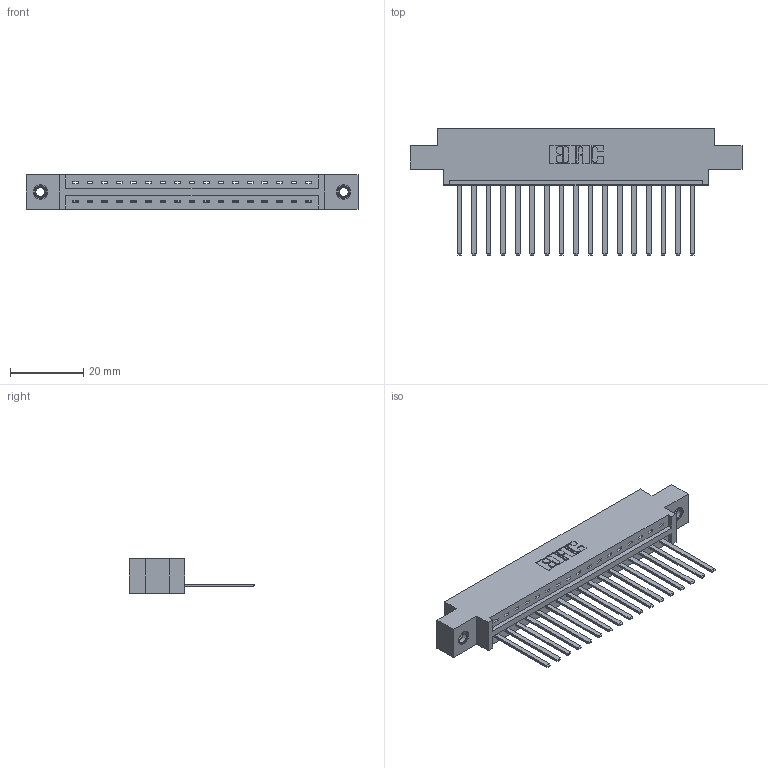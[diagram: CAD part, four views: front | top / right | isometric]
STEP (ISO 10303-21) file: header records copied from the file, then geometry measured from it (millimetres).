
FILE_DESCRIPTION (( 'STEP AP203' ), '1' );
FILE_NAME ('337-017-544-607.STEP', '2018-08-04T22:29:34', ( '' ), ( '' ), 'SwSTEP 2.0', 'SolidWorks 2016', '' );
FILE_SCHEMA (( 'CONFIG_CONTROL_DESIGN' ));
Length unit declared in the file: inch
Products named in the file (4): 337 Part_0.170 Offset - 0.156 Dia-TI; 345-292-001_345-293-144; 345-250-001_345-250-005-103; 337-017-544-607
Assembly tree (20 placements, depth 2):
  337-017-544-607
    337 Part_0.170 Offset - 0.156 Dia-TI
    345-292-001_345-293-144  x17
    345-250-001_345-250-005-103  x2
Bounding box: 90.37 x 34.3 x 9.4 mm (x, y, z)
Volume: 9145.8 mm3; surface area: 10097.2 mm2
Topology: 20 solids, 20 shells, 1130 faces, 3349 edges, 2202 vertices
Faces by surface type: plane 820, cylinder 294, cone 12, torus 4
Entity records: 17004 total; most frequent: CARTESIAN_POINT 2940, ORIENTED_EDGE 2886, DIRECTION 2555, EDGE_CURVE 1443, VECTOR 1299, LINE 1299, VERTEX_POINT 956, AXIS2_PLACEMENT_3D 628
